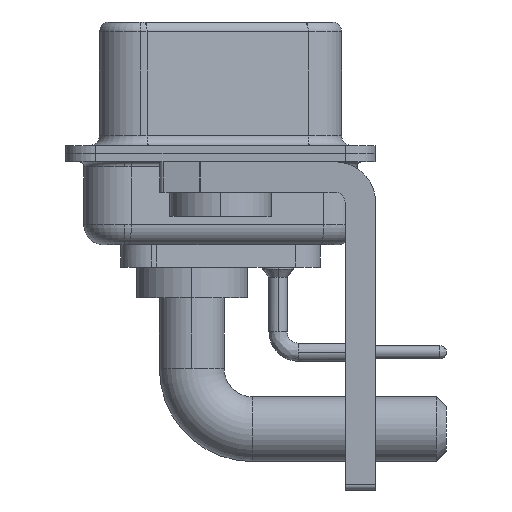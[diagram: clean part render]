
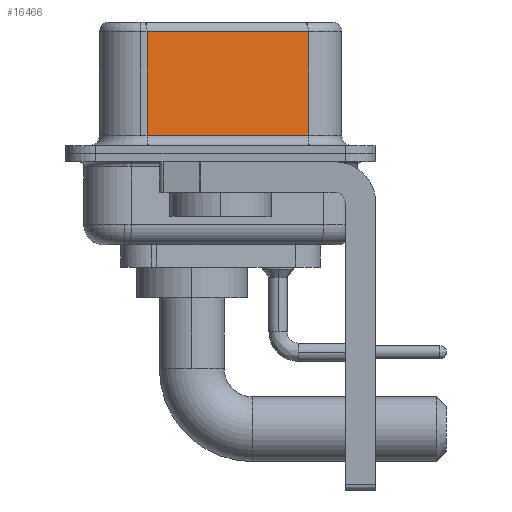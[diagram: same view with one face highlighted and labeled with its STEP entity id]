
A CAD part, left-side view. The second image highlights one B-rep face of the part: STEP entity #16466.
In plain terms, the highlighted planar face has unit normal (-0.985, -0.174, 0).
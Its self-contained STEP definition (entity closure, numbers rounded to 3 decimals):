
#644 = VERTEX_POINT ( 'NONE', #8358 ) ;
#1296 = CARTESIAN_POINT ( 'NONE',  ( 5.132, -4.322, 6.52 ) ) ;
#2000 = VECTOR ( 'NONE', #23437, 1000. ) ;
#3012 = DIRECTION ( 'NONE',  ( 0.985, 0.174, 0. ) ) ;
#3636 = CARTESIAN_POINT ( 'NONE',  ( 5.132, -4.322, 0.9 ) ) ;
#4827 = VECTOR ( 'NONE', #5755, 1000. ) ;
#5073 = EDGE_CURVE ( 'NONE', #8531, #16645, #16618, .T. ) ;
#5312 = VERTEX_POINT ( 'NONE', #15591 ) ;
#5755 = DIRECTION ( 'NONE',  ( 0.174, -0.985, 0. ) ) ;
#6168 = EDGE_CURVE ( 'NONE', #644, #5312, #21176, .T. ) ;
#6795 = FACE_OUTER_BOUND ( 'NONE', #13005, .T. ) ;
#7138 = VECTOR ( 'NONE', #24148, 1000. ) ;
#8358 = CARTESIAN_POINT ( 'NONE',  ( 3.73, 3.628, 6.02 ) ) ;
#8531 = VERTEX_POINT ( 'NONE', #12074 ) ;
#10663 = ORIENTED_EDGE ( 'NONE', *, *, #5073, .F. ) ;
#11517 = CARTESIAN_POINT ( 'NONE',  ( 3.73, 3.628, 6.52 ) ) ;
#12074 = CARTESIAN_POINT ( 'NONE',  ( 5.132, -4.322, 6.02 ) ) ;
#12989 = ORIENTED_EDGE ( 'NONE', *, *, #21109, .T. ) ;
#13005 = EDGE_LOOP ( 'NONE', ( #10663, #12989, #19127, #16189 ) ) ;
#13090 = DIRECTION ( 'NONE',  ( 0., 0., -1. ) ) ;
#14200 = DIRECTION ( 'NONE',  ( -0.174, 0.985, 0. ) ) ;
#14728 = CARTESIAN_POINT ( 'NONE',  ( 5.132, -4.322, 6.02 ) ) ;
#14853 = LINE ( 'NONE', #14728, #7138 ) ;
#15591 = CARTESIAN_POINT ( 'NONE',  ( 3.73, 3.628, 0.9 ) ) ;
#16097 = AXIS2_PLACEMENT_3D ( 'NONE', #23740, #3012, #14200 ) ;
#16189 = ORIENTED_EDGE ( 'NONE', *, *, #22129, .T. ) ;
#16466 = ADVANCED_FACE ( 'NONE', ( #6795 ), #18095, .F. ) ;
#16618 = LINE ( 'NONE', #1296, #23395 ) ;
#16645 = VERTEX_POINT ( 'NONE', #3636 ) ;
#18095 = PLANE ( 'NONE',  #16097 ) ;
#19127 = ORIENTED_EDGE ( 'NONE', *, *, #6168, .T. ) ;
#21109 = EDGE_CURVE ( 'NONE', #8531, #644, #14853, .T. ) ;
#21176 = LINE ( 'NONE', #11517, #2000 ) ;
#22129 = EDGE_CURVE ( 'NONE', #5312, #16645, #24708, .T. ) ;
#23395 = VECTOR ( 'NONE', #13090, 1000. ) ;
#23437 = DIRECTION ( 'NONE',  ( 0., 0., -1. ) ) ;
#23740 = CARTESIAN_POINT ( 'NONE',  ( 5.132, -4.322, 6.52 ) ) ;
#24148 = DIRECTION ( 'NONE',  ( -0.174, 0.985, 0. ) ) ;
#24456 = CARTESIAN_POINT ( 'NONE',  ( 5.132, -4.322, 0.9 ) ) ;
#24708 = LINE ( 'NONE', #24456, #4827 ) ;
